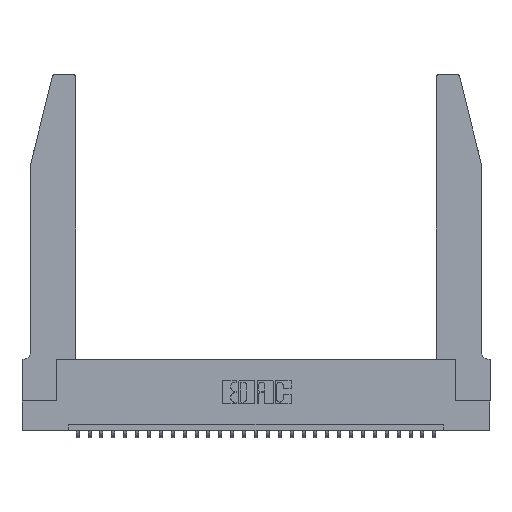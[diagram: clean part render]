
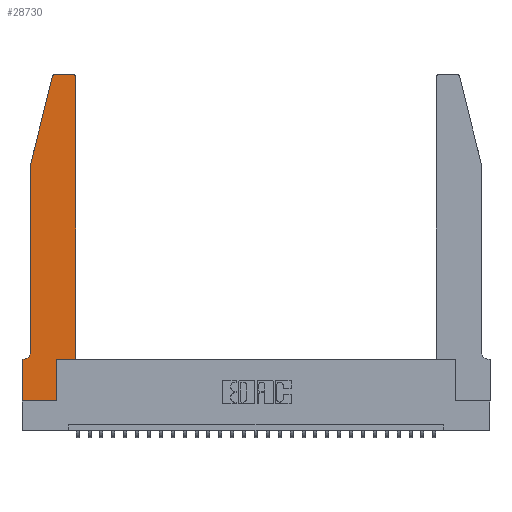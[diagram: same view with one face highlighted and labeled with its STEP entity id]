
A CAD part, top view. The second image highlights one B-rep face of the part: STEP entity #28730.
In plain terms, the highlighted planar face has unit normal (0, 0, 1).
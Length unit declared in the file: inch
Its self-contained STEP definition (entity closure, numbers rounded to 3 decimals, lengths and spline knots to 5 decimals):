
#290 = CARTESIAN_POINT ( 'NONE',  ( 0.4505, 0.35, 0.37 ) ) ;
#358 = EDGE_CURVE ( 'NONE', #27139, #24017, #4188, .T. ) ;
#462 = VECTOR ( 'NONE', #22765, 39.37008 ) ;
#1372 = CARTESIAN_POINT ( 'NONE',  ( 0., 0., 0.37 ) ) ;
#1439 = CARTESIAN_POINT ( 'NONE',  ( 0.0755, 2., 0.37 ) ) ;
#1495 = VECTOR ( 'NONE', #26088, 39.37008 ) ;
#2459 = EDGE_CURVE ( 'NONE', #7354, #5128, #25851, .T. ) ;
#3135 = VERTEX_POINT ( 'NONE', #27035 ) ;
#3275 = DIRECTION ( 'NONE',  ( 0., 0., 1. ) ) ;
#4188 = LINE ( 'NONE', #4983, #12367 ) ;
#4336 = CARTESIAN_POINT ( 'NONE',  ( 0.0755, 2., 0.37 ) ) ;
#4663 = ORIENTED_EDGE ( 'NONE', *, *, #20615, .T. ) ;
#4983 = CARTESIAN_POINT ( 'NONE',  ( 0.2865, 0.35, 0.37 ) ) ;
#5128 = VERTEX_POINT ( 'NONE', #14325 ) ;
#5345 = PLANE ( 'NONE',  #6910 ) ;
#5503 = LINE ( 'NONE', #7841, #12298 ) ;
#5928 = DIRECTION ( 'NONE',  ( -1., 0., 0. ) ) ;
#6041 = EDGE_CURVE ( 'NONE', #29586, #8845, #5503, .T. ) ;
#6602 = ORIENTED_EDGE ( 'NONE', *, *, #29333, .T. ) ;
#6605 = CIRCLE ( 'NONE', #14892, 0.03 ) ;
#6686 = CARTESIAN_POINT ( 'NONE',  ( 0.2865, 0.35, 0.37 ) ) ;
#6762 = CARTESIAN_POINT ( 'NONE',  ( 0.0755, 0.35, 0.37 ) ) ;
#6910 = AXIS2_PLACEMENT_3D ( 'NONE', #19148, #3275, #23727 ) ;
#7354 = VERTEX_POINT ( 'NONE', #8767 ) ;
#7616 = CARTESIAN_POINT ( 'NONE',  ( 0.4205, 2.72, 0.37 ) ) ;
#7667 = EDGE_LOOP ( 'NONE', ( #8210, #29361, #6602, #9951, #11537, #26014, #21740, #22341, #15969, #27883, #4663, #20111 ) ) ;
#7737 = VECTOR ( 'NONE', #16440, 39.37008 ) ;
#7834 = CARTESIAN_POINT ( 'NONE',  ( 0.4505, 0.35, 0.37 ) ) ;
#7841 = CARTESIAN_POINT ( 'NONE',  ( 0., 0., 0.37 ) ) ;
#8027 = VERTEX_POINT ( 'NONE', #16105 ) ;
#8210 = ORIENTED_EDGE ( 'NONE', *, *, #15512, .T. ) ;
#8528 = CARTESIAN_POINT ( 'NONE',  ( 0.4505, 0.35, 0.37 ) ) ;
#8676 = CARTESIAN_POINT ( 'NONE',  ( 0.25487, 2.72718, 0.37 ) ) ;
#8767 = CARTESIAN_POINT ( 'NONE',  ( 0.4505, 2.72, 0.37 ) ) ;
#8813 = LINE ( 'NONE', #290, #7737 ) ;
#8845 = VERTEX_POINT ( 'NONE', #15965 ) ;
#9500 = DIRECTION ( 'NONE',  ( 0., 1., 0. ) ) ;
#9696 = LINE ( 'NONE', #10233, #11447 ) ;
#9747 = EDGE_CURVE ( 'NONE', #3135, #8027, #14602, .T. ) ;
#9951 = ORIENTED_EDGE ( 'NONE', *, *, #16200, .T. ) ;
#10220 = DIRECTION ( 'NONE',  ( 0., -1., 0. ) ) ;
#10233 = CARTESIAN_POINT ( 'NONE',  ( 0.0755, 2., 0.37 ) ) ;
#11125 = DIRECTION ( 'NONE',  ( 0., 0., 1. ) ) ;
#11447 = VECTOR ( 'NONE', #16912, 39.37008 ) ;
#11537 = ORIENTED_EDGE ( 'NONE', *, *, #9747, .T. ) ;
#12298 = VECTOR ( 'NONE', #12325, 39.37008 ) ;
#12325 = DIRECTION ( 'NONE',  ( 0., -1., 0. ) ) ;
#12367 = VECTOR ( 'NONE', #9500, 39.37008 ) ;
#12525 = EDGE_CURVE ( 'NONE', #16669, #15217, #6605, .T. ) ;
#12538 = VERTEX_POINT ( 'NONE', #4336 ) ;
#13027 = DIRECTION ( 'NONE',  ( 0., 1., 0. ) ) ;
#14153 = LINE ( 'NONE', #1372, #23805 ) ;
#14325 = CARTESIAN_POINT ( 'NONE',  ( 0.4205, 2.75, 0.37 ) ) ;
#14602 = CIRCLE ( 'NONE', #20603, 0.07 ) ;
#14892 = AXIS2_PLACEMENT_3D ( 'NONE', #18033, #11125, #22521 ) ;
#15217 = VERTEX_POINT ( 'NONE', #8676 ) ;
#15512 = EDGE_CURVE ( 'NONE', #5128, #16669, #17543, .T. ) ;
#15673 = CARTESIAN_POINT ( 'NONE',  ( 0.2865, 0., 0.37 ) ) ;
#15965 = CARTESIAN_POINT ( 'NONE',  ( 0., 0., 0.37 ) ) ;
#15969 = ORIENTED_EDGE ( 'NONE', *, *, #358, .T. ) ;
#16105 = CARTESIAN_POINT ( 'NONE',  ( 0.0055, 0.35, 0.37 ) ) ;
#16200 = EDGE_CURVE ( 'NONE', #12538, #3135, #27189, .T. ) ;
#16440 = DIRECTION ( 'NONE',  ( 1., 0., 0. ) ) ;
#16669 = VERTEX_POINT ( 'NONE', #22052 ) ;
#16774 = DIRECTION ( 'NONE',  ( 1., 0., 0. ) ) ;
#16912 = DIRECTION ( 'NONE',  ( -0.239, -0.971, 0. ) ) ;
#17543 = LINE ( 'NONE', #20977, #1495 ) ;
#18033 = CARTESIAN_POINT ( 'NONE',  ( 0.284, 2.72, 0.37 ) ) ;
#18868 = VERTEX_POINT ( 'NONE', #7834 ) ;
#18891 = DIRECTION ( 'NONE',  ( 0., 0., 1. ) ) ;
#19027 = LINE ( 'NONE', #6762, #462 ) ;
#19148 = CARTESIAN_POINT ( 'NONE',  ( 0., 0.35, 0.37 ) ) ;
#20111 = ORIENTED_EDGE ( 'NONE', *, *, #2459, .T. ) ;
#20294 = EDGE_CURVE ( 'NONE', #24017, #18868, #8813, .T. ) ;
#20603 = AXIS2_PLACEMENT_3D ( 'NONE', #21831, #24026, #5928 ) ;
#20615 = EDGE_CURVE ( 'NONE', #18868, #7354, #20962, .T. ) ;
#20812 = FACE_OUTER_BOUND ( 'NONE', #7667, .T. ) ;
#20962 = LINE ( 'NONE', #8528, #29256 ) ;
#20977 = CARTESIAN_POINT ( 'NONE',  ( 0.2605, 2.75, 0.37 ) ) ;
#21740 = ORIENTED_EDGE ( 'NONE', *, *, #6041, .T. ) ;
#21831 = CARTESIAN_POINT ( 'NONE',  ( 0.0055, 0.42, 0.37 ) ) ;
#22052 = CARTESIAN_POINT ( 'NONE',  ( 0.284, 2.75, 0.37 ) ) ;
#22341 = ORIENTED_EDGE ( 'NONE', *, *, #26424, .T. ) ;
#22521 = DIRECTION ( 'NONE',  ( 1., 0., 0. ) ) ;
#22765 = DIRECTION ( 'NONE',  ( -1., 0., 0. ) ) ;
#23727 = DIRECTION ( 'NONE',  ( 1., 0., 0. ) ) ;
#23805 = VECTOR ( 'NONE', #26839, 39.37008 ) ;
#24017 = VERTEX_POINT ( 'NONE', #6686 ) ;
#24026 = DIRECTION ( 'NONE',  ( 0., 0., -1. ) ) ;
#25851 = CIRCLE ( 'NONE', #28975, 0.03 ) ;
#26014 = ORIENTED_EDGE ( 'NONE', *, *, #28459, .T. ) ;
#26088 = DIRECTION ( 'NONE',  ( -1., 0., 0. ) ) ;
#26424 = EDGE_CURVE ( 'NONE', #8845, #27139, #14153, .T. ) ;
#26839 = DIRECTION ( 'NONE',  ( 1., 0., 0. ) ) ;
#27035 = CARTESIAN_POINT ( 'NONE',  ( 0.0755, 0.42, 0.37 ) ) ;
#27139 = VERTEX_POINT ( 'NONE', #15673 ) ;
#27189 = LINE ( 'NONE', #1439, #29363 ) ;
#27408 = CARTESIAN_POINT ( 'NONE',  ( 0., 0.35, 0.37 ) ) ;
#27883 = ORIENTED_EDGE ( 'NONE', *, *, #20294, .T. ) ;
#28459 = EDGE_CURVE ( 'NONE', #8027, #29586, #19027, .T. ) ;
#28730 = ADVANCED_FACE ( 'NONE', ( #20812 ), #5345, .T. ) ;
#28975 = AXIS2_PLACEMENT_3D ( 'NONE', #7616, #18891, #16774 ) ;
#29256 = VECTOR ( 'NONE', #13027, 39.37008 ) ;
#29333 = EDGE_CURVE ( 'NONE', #15217, #12538, #9696, .T. ) ;
#29361 = ORIENTED_EDGE ( 'NONE', *, *, #12525, .T. ) ;
#29363 = VECTOR ( 'NONE', #10220, 39.37008 ) ;
#29586 = VERTEX_POINT ( 'NONE', #27408 ) ;
